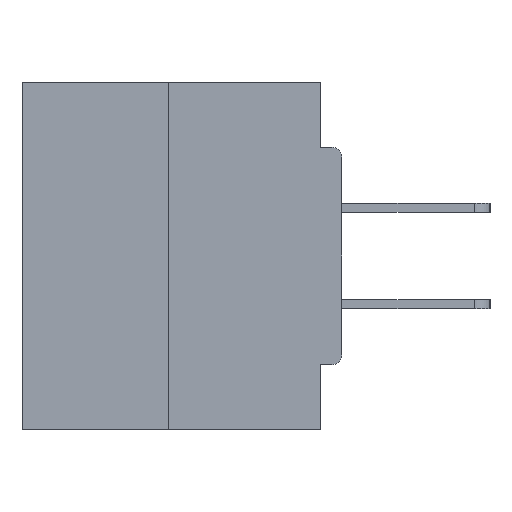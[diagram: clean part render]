
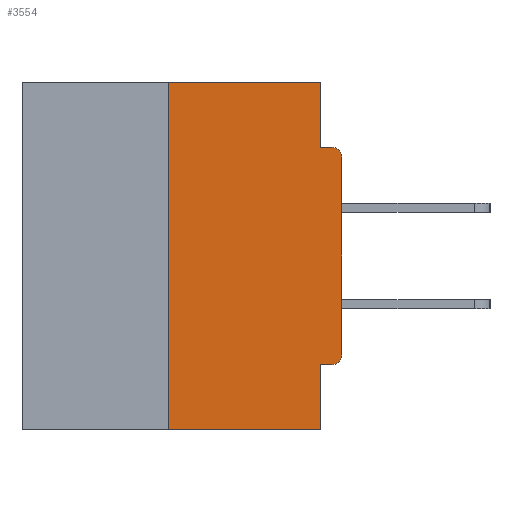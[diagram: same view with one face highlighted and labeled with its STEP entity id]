
A CAD part, left-side view. The second image highlights one B-rep face of the part: STEP entity #3554.
In plain terms, the highlighted planar face has unit normal (-1, 0, 0).
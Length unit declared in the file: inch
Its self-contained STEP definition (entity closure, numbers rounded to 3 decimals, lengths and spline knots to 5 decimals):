
#105 = EDGE_CURVE ( 'NONE', #27811, #30005, #28519, .T. ) ;
#1826 = DIRECTION ( 'NONE',  ( 0., 0., -1. ) ) ;
#1911 = VECTOR ( 'NONE', #28534, 39.37008 ) ;
#2706 = ORIENTED_EDGE ( 'NONE', *, *, #9393, .F. ) ;
#3554 = ADVANCED_FACE ( 'NONE', ( #9343 ), #30509, .F. ) ;
#4172 = LINE ( 'NONE', #6085, #27659 ) ;
#4577 = ORIENTED_EDGE ( 'NONE', *, *, #30629, .F. ) ;
#5848 = CARTESIAN_POINT ( 'NONE',  ( 0., 0.46, -0.5 ) ) ;
#6015 = CARTESIAN_POINT ( 'NONE',  ( 0., 0., 0. ) ) ;
#6031 = EDGE_CURVE ( 'NONE', #11551, #10042, #4172, .T. ) ;
#6085 = CARTESIAN_POINT ( 'NONE',  ( 0., 0., -0.0935 ) ) ;
#6372 = CIRCLE ( 'NONE', #21251, 0.015 ) ;
#6404 = CARTESIAN_POINT ( 'NONE',  ( 0., 0.46, 0. ) ) ;
#7817 = LINE ( 'NONE', #6015, #30971 ) ;
#7937 = CARTESIAN_POINT ( 'NONE',  ( 0., 0.25, 0. ) ) ;
#8397 = ORIENTED_EDGE ( 'NONE', *, *, #105, .F. ) ;
#8696 = CARTESIAN_POINT ( 'NONE',  ( 0., 0.015, -0.0935 ) ) ;
#8801 = EDGE_CURVE ( 'NONE', #11688, #29849, #18996, .T. ) ;
#9343 = FACE_OUTER_BOUND ( 'NONE', #16801, .T. ) ;
#9393 = EDGE_CURVE ( 'NONE', #16071, #27811, #30433, .T. ) ;
#10042 = VERTEX_POINT ( 'NONE', #8696 ) ;
#11416 = DIRECTION ( 'NONE',  ( 0., 0., -1. ) ) ;
#11551 = VERTEX_POINT ( 'NONE', #28489 ) ;
#11688 = VERTEX_POINT ( 'NONE', #29044 ) ;
#12418 = VECTOR ( 'NONE', #24900, 39.37008 ) ;
#12454 = ORIENTED_EDGE ( 'NONE', *, *, #26316, .T. ) ;
#12500 = DIRECTION ( 'NONE',  ( -1., 0., 0. ) ) ;
#12530 = CARTESIAN_POINT ( 'NONE',  ( 0., 0.031, 0. ) ) ;
#13211 = AXIS2_PLACEMENT_3D ( 'NONE', #22108, #12500, #19750 ) ;
#13320 = DIRECTION ( 'NONE',  ( 0., 0., -1. ) ) ;
#13398 = ORIENTED_EDGE ( 'NONE', *, *, #24545, .T. ) ;
#13790 = VERTEX_POINT ( 'NONE', #30849 ) ;
#13897 = CIRCLE ( 'NONE', #13211, 0.015 ) ;
#13969 = CARTESIAN_POINT ( 'NONE',  ( 0., 0.031, 0. ) ) ;
#14142 = CARTESIAN_POINT ( 'NONE',  ( 0., 0.031, -0.4065 ) ) ;
#16071 = VERTEX_POINT ( 'NONE', #16191 ) ;
#16191 = CARTESIAN_POINT ( 'NONE',  ( 0., 0.015, -0.4065 ) ) ;
#16209 = DIRECTION ( 'NONE',  ( -1., 0., 0. ) ) ;
#16638 = CARTESIAN_POINT ( 'NONE',  ( 0., 0., -0.4065 ) ) ;
#16801 = EDGE_LOOP ( 'NONE', ( #18955, #20429, #30528, #8397, #2706, #12454, #31388, #13398, #21587, #4577 ) ) ;
#17270 = VECTOR ( 'NONE', #28860, 39.37008 ) ;
#17585 = EDGE_CURVE ( 'NONE', #29849, #27145, #22847, .T. ) ;
#17977 = EDGE_CURVE ( 'NONE', #13790, #20621, #7817, .T. ) ;
#18180 = CARTESIAN_POINT ( 'NONE',  ( 0., 0.46, 0. ) ) ;
#18414 = DIRECTION ( 'NONE',  ( 1., 0., 0. ) ) ;
#18468 = DIRECTION ( 'NONE',  ( 0., -1., 0. ) ) ;
#18504 = DIRECTION ( 'NONE',  ( 0., 0., 1. ) ) ;
#18642 = VECTOR ( 'NONE', #31098, 39.37008 ) ;
#18926 = CARTESIAN_POINT ( 'NONE',  ( 0., 0.015, -0.1085 ) ) ;
#18955 = ORIENTED_EDGE ( 'NONE', *, *, #17585, .F. ) ;
#18996 = LINE ( 'NONE', #20027, #12418 ) ;
#19750 = DIRECTION ( 'NONE',  ( 0., 0., -1. ) ) ;
#20027 = CARTESIAN_POINT ( 'NONE',  ( 0., 0.25, 0. ) ) ;
#20429 = ORIENTED_EDGE ( 'NONE', *, *, #8801, .F. ) ;
#20621 = VERTEX_POINT ( 'NONE', #23907 ) ;
#20949 = VECTOR ( 'NONE', #23188, 39.37008 ) ;
#21251 = AXIS2_PLACEMENT_3D ( 'NONE', #18926, #16209, #1826 ) ;
#21587 = ORIENTED_EDGE ( 'NONE', *, *, #6031, .F. ) ;
#21784 = EDGE_CURVE ( 'NONE', #11688, #30005, #31062, .T. ) ;
#22108 = CARTESIAN_POINT ( 'NONE',  ( 0., 0.015, -0.3915 ) ) ;
#22293 = VECTOR ( 'NONE', #11416, 39.37008 ) ;
#22847 = LINE ( 'NONE', #6404, #18642 ) ;
#23188 = DIRECTION ( 'NONE',  ( 0., -1., 0. ) ) ;
#23907 = CARTESIAN_POINT ( 'NONE',  ( 0., 0., -0.1085 ) ) ;
#24545 = EDGE_CURVE ( 'NONE', #20621, #10042, #6372, .T. ) ;
#24725 = CARTESIAN_POINT ( 'NONE',  ( 0., 0.031, -0.5 ) ) ;
#24900 = DIRECTION ( 'NONE',  ( 0., 0., 1. ) ) ;
#25453 = AXIS2_PLACEMENT_3D ( 'NONE', #18180, #18414, #13320 ) ;
#26316 = EDGE_CURVE ( 'NONE', #16071, #13790, #13897, .T. ) ;
#27145 = VERTEX_POINT ( 'NONE', #12530 ) ;
#27659 = VECTOR ( 'NONE', #18468, 39.37008 ) ;
#27811 = VERTEX_POINT ( 'NONE', #14142 ) ;
#28489 = CARTESIAN_POINT ( 'NONE',  ( 0., 0.031, -0.0935 ) ) ;
#28519 = LINE ( 'NONE', #28639, #1911 ) ;
#28534 = DIRECTION ( 'NONE',  ( 0., 0., -1. ) ) ;
#28639 = CARTESIAN_POINT ( 'NONE',  ( 0., 0.031, -0.5 ) ) ;
#28860 = DIRECTION ( 'NONE',  ( 0., 1., 0. ) ) ;
#29044 = CARTESIAN_POINT ( 'NONE',  ( 0., 0.25, -0.5 ) ) ;
#29667 = LINE ( 'NONE', #13969, #22293 ) ;
#29849 = VERTEX_POINT ( 'NONE', #7937 ) ;
#30005 = VERTEX_POINT ( 'NONE', #24725 ) ;
#30433 = LINE ( 'NONE', #16638, #17270 ) ;
#30509 = PLANE ( 'NONE',  #25453 ) ;
#30528 = ORIENTED_EDGE ( 'NONE', *, *, #21784, .T. ) ;
#30629 = EDGE_CURVE ( 'NONE', #27145, #11551, #29667, .T. ) ;
#30849 = CARTESIAN_POINT ( 'NONE',  ( 0., 0., -0.3915 ) ) ;
#30971 = VECTOR ( 'NONE', #18504, 39.37008 ) ;
#31062 = LINE ( 'NONE', #5848, #20949 ) ;
#31098 = DIRECTION ( 'NONE',  ( 0., -1., 0. ) ) ;
#31388 = ORIENTED_EDGE ( 'NONE', *, *, #17977, .T. ) ;
